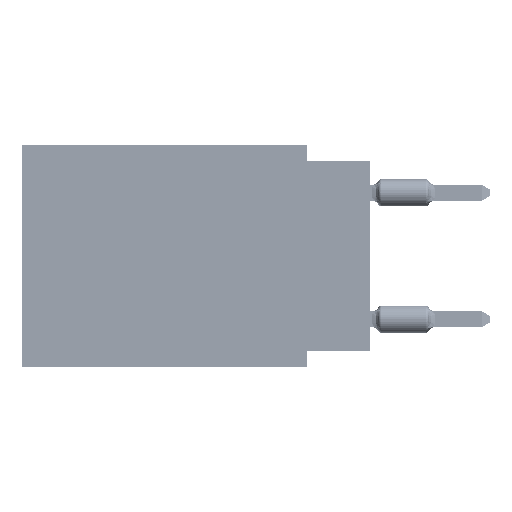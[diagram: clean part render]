
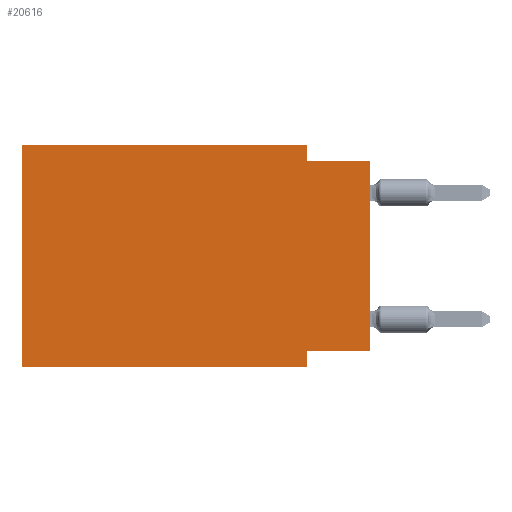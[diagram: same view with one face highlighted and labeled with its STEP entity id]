
A CAD part, left-side view. The second image highlights one B-rep face of the part: STEP entity #20616.
In plain terms, the highlighted planar face has unit normal (-1, 0, 0).
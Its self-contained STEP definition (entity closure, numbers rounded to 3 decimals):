
#1275 = CARTESIAN_POINT ( 'NONE',  ( 0., 0., -0.635 ) ) ;
#4202 = VERTEX_POINT ( 'NONE', #71446 ) ;
#4646 = VERTEX_POINT ( 'NONE', #7045 ) ;
#5726 = VECTOR ( 'NONE', #18749, 1000. ) ;
#6222 = VECTOR ( 'NONE', #74163, 1000. ) ;
#7045 = CARTESIAN_POINT ( 'NONE',  ( 0., 2.54, 0. ) ) ;
#8240 = VECTOR ( 'NONE', #69758, 1000. ) ;
#10667 = VERTEX_POINT ( 'NONE', #20260 ) ;
#11580 = DIRECTION ( 'NONE',  ( 0., -1., 0. ) ) ;
#11792 = DIRECTION ( 'NONE',  ( 0., 0., 1. ) ) ;
#11999 = DIRECTION ( 'NONE',  ( 1., 0., 0. ) ) ;
#13530 = EDGE_CURVE ( 'NONE', #74995, #23680, #28103, .T. ) ;
#15026 = EDGE_CURVE ( 'NONE', #46162, #4646, #29074, .T. ) ;
#15062 = CARTESIAN_POINT ( 'NONE',  ( 0., 2.54, 0. ) ) ;
#16470 = LINE ( 'NONE', #28777, #54287 ) ;
#17975 = PLANE ( 'NONE',  #25900 ) ;
#18358 = DIRECTION ( 'NONE',  ( 0., 0., -1. ) ) ;
#18749 = DIRECTION ( 'NONE',  ( 0., -1., 0. ) ) ;
#20260 = CARTESIAN_POINT ( 'NONE',  ( 0., 0., -8.255 ) ) ;
#20577 = CARTESIAN_POINT ( 'NONE',  ( 0., 2.54, -8.89 ) ) ;
#20616 = ADVANCED_FACE ( 'NONE', ( #36217 ), #17975, .F. ) ;
#21053 = VECTOR ( 'NONE', #11580, 1000. ) ;
#22942 = VERTEX_POINT ( 'NONE', #72659 ) ;
#23680 = VERTEX_POINT ( 'NONE', #60593 ) ;
#25837 = EDGE_CURVE ( 'NONE', #53629, #22942, #38185, .T. ) ;
#25900 = AXIS2_PLACEMENT_3D ( 'NONE', #48924, #11999, #18358 ) ;
#26890 = VECTOR ( 'NONE', #75342, 1000. ) ;
#28103 = LINE ( 'NONE', #20577, #8240 ) ;
#28777 = CARTESIAN_POINT ( 'NONE',  ( 0., 13.97, 0. ) ) ;
#29074 = LINE ( 'NONE', #60383, #21053 ) ;
#29661 = CARTESIAN_POINT ( 'NONE',  ( 0., 0., 0. ) ) ;
#29970 = VECTOR ( 'NONE', #11792, 1000. ) ;
#30066 = LINE ( 'NONE', #29661, #29970 ) ;
#32765 = ORIENTED_EDGE ( 'NONE', *, *, #13530, .F. ) ;
#32928 = CARTESIAN_POINT ( 'NONE',  ( 0., 0., -8.255 ) ) ;
#32976 = ORIENTED_EDGE ( 'NONE', *, *, #15026, .F. ) ;
#33715 = DIRECTION ( 'NONE',  ( 0., -1., 0. ) ) ;
#33951 = DIRECTION ( 'NONE',  ( 0., 0., 1. ) ) ;
#36217 = FACE_OUTER_BOUND ( 'NONE', #64564, .T. ) ;
#37153 = EDGE_CURVE ( 'NONE', #4646, #53629, #56730, .T. ) ;
#38185 = LINE ( 'NONE', #1275, #5726 ) ;
#40593 = CARTESIAN_POINT ( 'NONE',  ( 0., 13.97, 0. ) ) ;
#43190 = ORIENTED_EDGE ( 'NONE', *, *, #65930, .T. ) ;
#44840 = LINE ( 'NONE', #32928, #26890 ) ;
#45267 = ORIENTED_EDGE ( 'NONE', *, *, #69288, .F. ) ;
#46117 = CARTESIAN_POINT ( 'NONE',  ( 0., 2.54, -0.635 ) ) ;
#46162 = VERTEX_POINT ( 'NONE', #40593 ) ;
#48924 = CARTESIAN_POINT ( 'NONE',  ( 0., 13.97, 0. ) ) ;
#53629 = VERTEX_POINT ( 'NONE', #46117 ) ;
#54287 = VECTOR ( 'NONE', #33951, 1000. ) ;
#56730 = LINE ( 'NONE', #15062, #6222 ) ;
#56939 = EDGE_CURVE ( 'NONE', #10667, #22942, #30066, .T. ) ;
#60383 = CARTESIAN_POINT ( 'NONE',  ( 0., 13.97, 0. ) ) ;
#60593 = CARTESIAN_POINT ( 'NONE',  ( 0., 2.54, -8.89 ) ) ;
#63005 = ORIENTED_EDGE ( 'NONE', *, *, #25837, .F. ) ;
#63855 = LINE ( 'NONE', #69027, #67474 ) ;
#64564 = EDGE_LOOP ( 'NONE', ( #72002, #63005, #75593, #32976, #65567, #43190, #32765, #45267 ) ) ;
#65066 = CARTESIAN_POINT ( 'NONE',  ( 0., 2.54, -8.255 ) ) ;
#65567 = ORIENTED_EDGE ( 'NONE', *, *, #78158, .F. ) ;
#65930 = EDGE_CURVE ( 'NONE', #4202, #23680, #63855, .T. ) ;
#67474 = VECTOR ( 'NONE', #33715, 1000. ) ;
#69027 = CARTESIAN_POINT ( 'NONE',  ( 0., 13.97, -8.89 ) ) ;
#69288 = EDGE_CURVE ( 'NONE', #10667, #74995, #44840, .T. ) ;
#69758 = DIRECTION ( 'NONE',  ( 0., 0., -1. ) ) ;
#71446 = CARTESIAN_POINT ( 'NONE',  ( 0., 13.97, -8.89 ) ) ;
#72002 = ORIENTED_EDGE ( 'NONE', *, *, #56939, .T. ) ;
#72659 = CARTESIAN_POINT ( 'NONE',  ( 0., 0., -0.635 ) ) ;
#74163 = DIRECTION ( 'NONE',  ( 0., 0., -1. ) ) ;
#74995 = VERTEX_POINT ( 'NONE', #65066 ) ;
#75342 = DIRECTION ( 'NONE',  ( 0., 1., 0. ) ) ;
#75593 = ORIENTED_EDGE ( 'NONE', *, *, #37153, .F. ) ;
#78158 = EDGE_CURVE ( 'NONE', #4202, #46162, #16470, .T. ) ;
